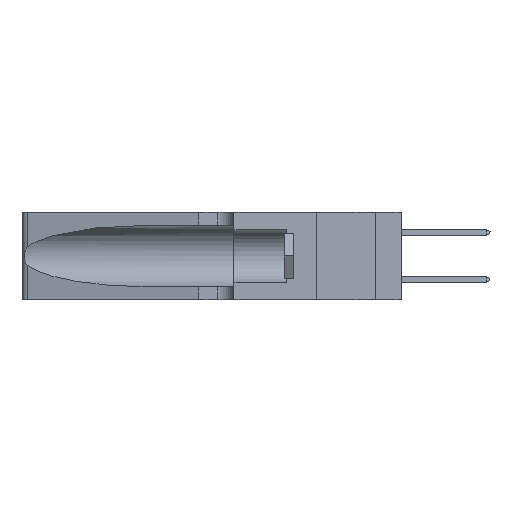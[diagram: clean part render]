
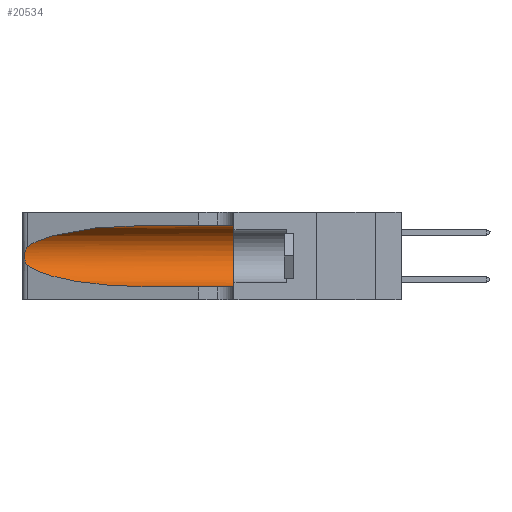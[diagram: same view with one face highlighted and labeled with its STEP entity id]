
A CAD part, left-side view. The second image highlights one B-rep face of the part: STEP entity #20534.
In plain terms, the highlighted cylindrical face has radius 3.308 mm (diameter 6.617 mm), a partial arc.
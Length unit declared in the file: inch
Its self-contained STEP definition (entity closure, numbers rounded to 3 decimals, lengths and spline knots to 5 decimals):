
#1437 =( BOUNDED_CURVE ( )  B_SPLINE_CURVE ( 3, ( #8437, #39740, #22473, #1550 ),
 .UNSPECIFIED., .F., .F. ) 
 B_SPLINE_CURVE_WITH_KNOTS ( ( 4, 4 ),
 ( 1.5708, 2.84003 ),
 .UNSPECIFIED. ) 
 CURVE ( )  GEOMETRIC_REPRESENTATION_ITEM ( )  RATIONAL_B_SPLINE_CURVE ( ( 1., 0.87, 0.87, 1. ) ) 
 REPRESENTATION_ITEM ( '' )  );
#1550 = CARTESIAN_POINT ( 'NONE',  ( 0.25487, 1.22718, 0.22369 ) ) ;
#2053 = DIRECTION ( 'NONE',  ( 0., 1., 0. ) ) ;
#2621 = VERTEX_POINT ( 'NONE', #36896 ) ;
#2956 = CARTESIAN_POINT ( 'NONE',  ( 0.1305, 1.61858, 0.31525 ) ) ;
#3733 = EDGE_CURVE ( 'NONE', #26317, #4989, #37496, .T. ) ;
#3962 = CARTESIAN_POINT ( 'NONE',  ( 0.25787, 1.23484, 0.2124 ) ) ;
#4989 = VERTEX_POINT ( 'NONE', #35249 ) ;
#5733 = ORIENTED_EDGE ( 'NONE', *, *, #34120, .T. ) ;
#6070 = B_SPLINE_CURVE_WITH_KNOTS ( 'NONE', 3,
 ( #42090, #17843, #24857, #3962, #28336, #7483, #31803, #10994, #35308, #14493, #38787, #17999, #42237, #21474 ),
 .UNSPECIFIED., .F., .F.,
 ( 4, 2, 2, 2, 2, 2, 4 ),
 ( 0., 0.00027, 0.00053, 0.00107, 0.0016, 0.00187, 0.00214 ),
 .UNSPECIFIED. ) ;
#6479 = DIRECTION ( 'NONE',  ( 0., -1., 0. ) ) ;
#6489 = CARTESIAN_POINT ( 'NONE',  ( 0.1305, 0.72297, 0.05475 ) ) ;
#6490 = VECTOR ( 'NONE', #6479, 39.37008 ) ;
#7137 = CARTESIAN_POINT ( 'NONE',  ( 0.1305, 1.61858, 0.185 ) ) ;
#7483 = CARTESIAN_POINT ( 'NONE',  ( 0.26018, 1.23835, 0.19895 ) ) ;
#8437 = CARTESIAN_POINT ( 'NONE',  ( 0.1305, 0.72297, 0.31525 ) ) ;
#10994 = CARTESIAN_POINT ( 'NONE',  ( 0.26075, 1.23896, 0.178 ) ) ;
#11496 = CARTESIAN_POINT ( 'NONE',  ( 0.1305, 1.61858, 0.05475 ) ) ;
#13373 = CARTESIAN_POINT ( 'NONE',  ( 0.25487, 1.22718, 0.14631 ) ) ;
#14035 = CARTESIAN_POINT ( 'NONE',  ( 0.25487, 1.22718, 0.22369 ) ) ;
#14147 = DIRECTION ( 'NONE',  ( 0., -1., 0. ) ) ;
#14493 = CARTESIAN_POINT ( 'NONE',  ( 0.25856, 1.23593, 0.16098 ) ) ;
#15760 = LINE ( 'NONE', #2956, #6490 ) ;
#16179 = FACE_OUTER_BOUND ( 'NONE', #27910, .T. ) ;
#16696 = ORIENTED_EDGE ( 'NONE', *, *, #40118, .T. ) ;
#17638 = DIRECTION ( 'NONE',  ( 0., 0., -1. ) ) ;
#17843 = CARTESIAN_POINT ( 'NONE',  ( 0.25555, 1.22994, 0.2215 ) ) ;
#17999 = CARTESIAN_POINT ( 'NONE',  ( 0.25639, 1.23186, 0.15144 ) ) ;
#20534 = ADVANCED_FACE ( 'NONE', ( #16179 ), #41643, .F. ) ;
#21178 = VECTOR ( 'NONE', #35794, 39.37008 ) ;
#21474 = CARTESIAN_POINT ( 'NONE',  ( 0.25487, 1.22718, 0.14631 ) ) ;
#21926 = VERTEX_POINT ( 'NONE', #14035 ) ;
#22473 = CARTESIAN_POINT ( 'NONE',  ( 0.2373, 1.15595, 0.28018 ) ) ;
#22964 = CARTESIAN_POINT ( 'NONE',  ( 0.1305, 0.35, 0.185 ) ) ;
#23262 = ORIENTED_EDGE ( 'NONE', *, *, #3733, .T. ) ;
#23827 = ORIENTED_EDGE ( 'NONE', *, *, #29511, .F. ) ;
#23873 = CARTESIAN_POINT ( 'NONE',  ( 0.2373, 1.15595, 0.08982 ) ) ;
#24857 = CARTESIAN_POINT ( 'NONE',  ( 0.25639, 1.23184, 0.21858 ) ) ;
#26317 = VERTEX_POINT ( 'NONE', #41629 ) ;
#26458 = DIRECTION ( 'NONE',  ( 0., 0., 1. ) ) ;
#26649 = VERTEX_POINT ( 'NONE', #39979 ) ;
#27000 = ORIENTED_EDGE ( 'NONE', *, *, #28358, .T. ) ;
#27346 = CARTESIAN_POINT ( 'NONE',  ( 0.18966, 0.96281, 0.05475 ) ) ;
#27910 = EDGE_LOOP ( 'NONE', ( #5733, #27000, #16696, #23262, #36841, #23827 ) ) ;
#28336 = CARTESIAN_POINT ( 'NONE',  ( 0.25854, 1.2359, 0.20912 ) ) ;
#28358 = EDGE_CURVE ( 'NONE', #21926, #26649, #6070, .T. ) ;
#28570 = AXIS2_PLACEMENT_3D ( 'NONE', #22964, #2053, #26458 ) ;
#29511 = EDGE_CURVE ( 'NONE', #39022, #2621, #15760, .T. ) ;
#31583 = EDGE_CURVE ( 'NONE', #2621, #4989, #37126, .T. ) ;
#31803 = CARTESIAN_POINT ( 'NONE',  ( 0.26075, 1.23896, 0.19203 ) ) ;
#33082 =( BOUNDED_CURVE ( )  B_SPLINE_CURVE ( 3, ( #13373, #23873, #27346, #6489 ),
 .UNSPECIFIED., .F., .T. ) 
 B_SPLINE_CURVE_WITH_KNOTS ( ( 4, 4 ),
 ( 3.44316, 4.71239 ),
 .UNSPECIFIED. ) 
 CURVE ( )  GEOMETRIC_REPRESENTATION_ITEM ( )  RATIONAL_B_SPLINE_CURVE ( ( 1., 0.87, 0.87, 1. ) ) 
 REPRESENTATION_ITEM ( '' )  );
#33150 = AXIS2_PLACEMENT_3D ( 'NONE', #7137, #14147, #17638 ) ;
#34120 = EDGE_CURVE ( 'NONE', #39022, #21926, #1437, .T. ) ;
#35249 = CARTESIAN_POINT ( 'NONE',  ( 0.1305, 0.35, 0.05475 ) ) ;
#35308 = CARTESIAN_POINT ( 'NONE',  ( 0.26017, 1.23833, 0.17102 ) ) ;
#35794 = DIRECTION ( 'NONE',  ( 0., -1., 0. ) ) ;
#36841 = ORIENTED_EDGE ( 'NONE', *, *, #31583, .F. ) ;
#36896 = CARTESIAN_POINT ( 'NONE',  ( 0.1305, 0.35, 0.31525 ) ) ;
#37126 = CIRCLE ( 'NONE', #28570, 0.13025 ) ;
#37496 = LINE ( 'NONE', #11496, #21178 ) ;
#38787 = CARTESIAN_POINT ( 'NONE',  ( 0.25789, 1.23486, 0.15765 ) ) ;
#39022 = VERTEX_POINT ( 'NONE', #39094 ) ;
#39094 = CARTESIAN_POINT ( 'NONE',  ( 0.1305, 0.72297, 0.31525 ) ) ;
#39740 = CARTESIAN_POINT ( 'NONE',  ( 0.18966, 0.96281, 0.31525 ) ) ;
#39979 = CARTESIAN_POINT ( 'NONE',  ( 0.25487, 1.22718, 0.14631 ) ) ;
#40118 = EDGE_CURVE ( 'NONE', #26649, #26317, #33082, .T. ) ;
#41629 = CARTESIAN_POINT ( 'NONE',  ( 0.1305, 0.72297, 0.05475 ) ) ;
#41643 = CYLINDRICAL_SURFACE ( 'NONE', #33150, 0.13025 ) ;
#42090 = CARTESIAN_POINT ( 'NONE',  ( 0.25487, 1.22718, 0.22369 ) ) ;
#42237 = CARTESIAN_POINT ( 'NONE',  ( 0.25555, 1.22993, 0.14849 ) ) ;
